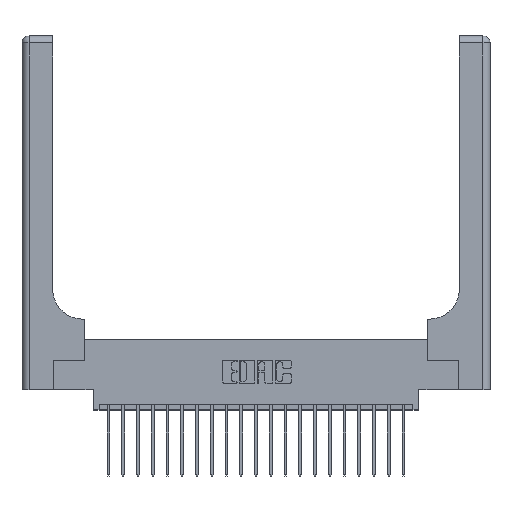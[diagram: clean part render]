
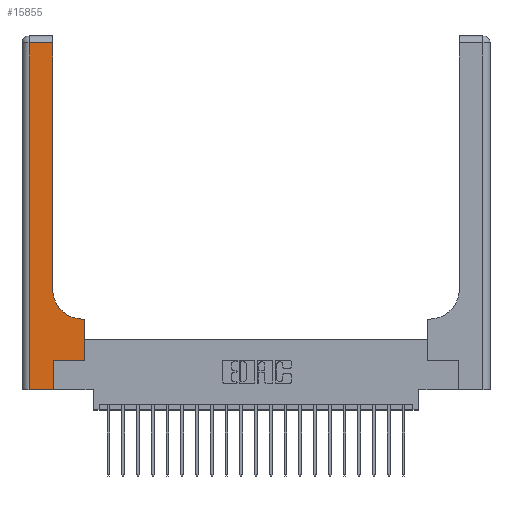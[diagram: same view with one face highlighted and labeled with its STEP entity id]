
A CAD part, top view. The second image highlights one B-rep face of the part: STEP entity #15855.
In plain terms, the highlighted planar face has unit normal (0, 0, 1).
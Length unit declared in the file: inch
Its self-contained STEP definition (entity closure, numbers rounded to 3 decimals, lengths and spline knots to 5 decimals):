
#29 = PLANE ( 'NONE',  #20371 ) ;
#299 = ORIENTED_EDGE ( 'NONE', *, *, #3143, .T. ) ;
#366 = FACE_OUTER_BOUND ( 'NONE', #4460, .T. ) ;
#551 = CARTESIAN_POINT ( 'NONE',  ( 0.51, 0.6, 0.37 ) ) ;
#690 = CARTESIAN_POINT ( 'NONE',  ( 0.265, 0., 0.37 ) ) ;
#1036 = EDGE_CURVE ( 'NONE', #14744, #18970, #10677, .T. ) ;
#1066 = CARTESIAN_POINT ( 'NONE',  ( 0.528, 0.25, 0.37 ) ) ;
#1901 = LINE ( 'NONE', #18936, #17615 ) ;
#1987 = LINE ( 'NONE', #22296, #10452 ) ;
#2389 = VERTEX_POINT ( 'NONE', #3256 ) ;
#2517 = ORIENTED_EDGE ( 'NONE', *, *, #4937, .T. ) ;
#2646 = ORIENTED_EDGE ( 'NONE', *, *, #11078, .T. ) ;
#3143 = EDGE_CURVE ( 'NONE', #7484, #9761, #21670, .T. ) ;
#3256 = CARTESIAN_POINT ( 'NONE',  ( 0.26, 2.94, 0.37 ) ) ;
#3376 = ORIENTED_EDGE ( 'NONE', *, *, #1036, .T. ) ;
#3458 = CARTESIAN_POINT ( 'NONE',  ( 0.265, 0.25, 0.37 ) ) ;
#3820 = EDGE_CURVE ( 'NONE', #18970, #9132, #1901, .T. ) ;
#4460 = EDGE_LOOP ( 'NONE', ( #7881, #10963, #5643, #299, #13958, #3376, #6700, #2646, #2517 ) ) ;
#4511 = CARTESIAN_POINT ( 'NONE',  ( 0.06, 0., 0.37 ) ) ;
#4746 = VERTEX_POINT ( 'NONE', #10046 ) ;
#4937 = EDGE_CURVE ( 'NONE', #7326, #4746, #17936, .T. ) ;
#5256 = DIRECTION ( 'NONE',  ( 0., 0., -1. ) ) ;
#5475 = DIRECTION ( 'NONE',  ( 1., 0., 0. ) ) ;
#5643 = ORIENTED_EDGE ( 'NONE', *, *, #9088, .T. ) ;
#5793 = CARTESIAN_POINT ( 'NONE',  ( 0.06, 2.94, 0.37 ) ) ;
#6700 = ORIENTED_EDGE ( 'NONE', *, *, #3820, .T. ) ;
#7108 = DIRECTION ( 'NONE',  ( 0., 1., 0. ) ) ;
#7326 = VERTEX_POINT ( 'NONE', #551 ) ;
#7484 = VERTEX_POINT ( 'NONE', #4511 ) ;
#7627 = VECTOR ( 'NONE', #19676, 39.37008 ) ;
#7670 = CARTESIAN_POINT ( 'NONE',  ( 0.51, 0.85, 0.37 ) ) ;
#7865 = DIRECTION ( 'NONE',  ( -1., 0., 0. ) ) ;
#7881 = ORIENTED_EDGE ( 'NONE', *, *, #9233, .T. ) ;
#8821 = VECTOR ( 'NONE', #7865, 39.37008 ) ;
#9088 = EDGE_CURVE ( 'NONE', #14943, #7484, #1987, .T. ) ;
#9132 = VERTEX_POINT ( 'NONE', #19230 ) ;
#9222 = VECTOR ( 'NONE', #22282, 39.37008 ) ;
#9233 = EDGE_CURVE ( 'NONE', #4746, #2389, #21489, .T. ) ;
#9761 = VERTEX_POINT ( 'NONE', #690 ) ;
#9802 = DIRECTION ( 'NONE',  ( 0., 0., -1. ) ) ;
#10046 = CARTESIAN_POINT ( 'NONE',  ( 0.26, 0.85, 0.37 ) ) ;
#10452 = VECTOR ( 'NONE', #14048, 39.37008 ) ;
#10553 = LINE ( 'NONE', #16961, #9222 ) ;
#10677 = LINE ( 'NONE', #3458, #20656 ) ;
#10963 = ORIENTED_EDGE ( 'NONE', *, *, #16406, .T. ) ;
#11078 = EDGE_CURVE ( 'NONE', #9132, #7326, #14108, .T. ) ;
#11393 = DIRECTION ( 'NONE',  ( 1., 0., 0. ) ) ;
#11886 = DIRECTION ( 'NONE',  ( 1., 0., 0. ) ) ;
#12873 = CARTESIAN_POINT ( 'NONE',  ( 0.26, 0.6, 0.37 ) ) ;
#13813 = CARTESIAN_POINT ( 'NONE',  ( 0., 3., 0.37 ) ) ;
#13958 = ORIENTED_EDGE ( 'NONE', *, *, #17932, .T. ) ;
#14048 = DIRECTION ( 'NONE',  ( 0., -1., 0. ) ) ;
#14108 = LINE ( 'NONE', #12873, #14109 ) ;
#14109 = VECTOR ( 'NONE', #21002, 39.37008 ) ;
#14744 = VERTEX_POINT ( 'NONE', #17718 ) ;
#14943 = VERTEX_POINT ( 'NONE', #5793 ) ;
#15855 = ADVANCED_FACE ( 'NONE', ( #366 ), #29, .F. ) ;
#16281 = CARTESIAN_POINT ( 'NONE',  ( 0.26, 3., 0.37 ) ) ;
#16406 = EDGE_CURVE ( 'NONE', #2389, #14943, #16627, .T. ) ;
#16627 = LINE ( 'NONE', #21600, #8821 ) ;
#16961 = CARTESIAN_POINT ( 'NONE',  ( 0.265, 0., 0.37 ) ) ;
#17615 = VECTOR ( 'NONE', #7108, 39.37008 ) ;
#17718 = CARTESIAN_POINT ( 'NONE',  ( 0.265, 0.25, 0.37 ) ) ;
#17932 = EDGE_CURVE ( 'NONE', #9761, #14744, #10553, .T. ) ;
#17936 = CIRCLE ( 'NONE', #20055, 0.25 ) ;
#18936 = CARTESIAN_POINT ( 'NONE',  ( 0.528, 0.25, 0.37 ) ) ;
#18970 = VERTEX_POINT ( 'NONE', #1066 ) ;
#19230 = CARTESIAN_POINT ( 'NONE',  ( 0.528, 0.6, 0.37 ) ) ;
#19676 = DIRECTION ( 'NONE',  ( 0., 1., 0. ) ) ;
#20055 = AXIS2_PLACEMENT_3D ( 'NONE', #7670, #9802, #11393 ) ;
#20371 = AXIS2_PLACEMENT_3D ( 'NONE', #13813, #5256, #20706 ) ;
#20436 = VECTOR ( 'NONE', #11886, 39.37008 ) ;
#20656 = VECTOR ( 'NONE', #5475, 39.37008 ) ;
#20706 = DIRECTION ( 'NONE',  ( -1., 0., 0. ) ) ;
#21002 = DIRECTION ( 'NONE',  ( -1., 0., 0. ) ) ;
#21489 = LINE ( 'NONE', #16281, #7627 ) ;
#21600 = CARTESIAN_POINT ( 'NONE',  ( 0., 2.94, 0.37 ) ) ;
#21670 = LINE ( 'NONE', #21793, #20436 ) ;
#21793 = CARTESIAN_POINT ( 'NONE',  ( 0., 0., 0.37 ) ) ;
#22282 = DIRECTION ( 'NONE',  ( 0., 1., 0. ) ) ;
#22296 = CARTESIAN_POINT ( 'NONE',  ( 0.06, 3., 0.37 ) ) ;
